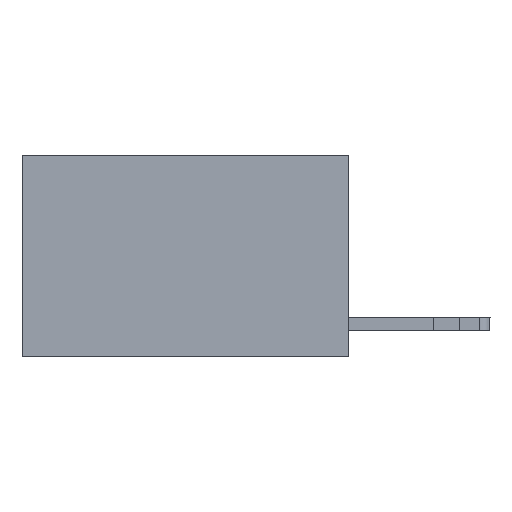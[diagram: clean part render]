
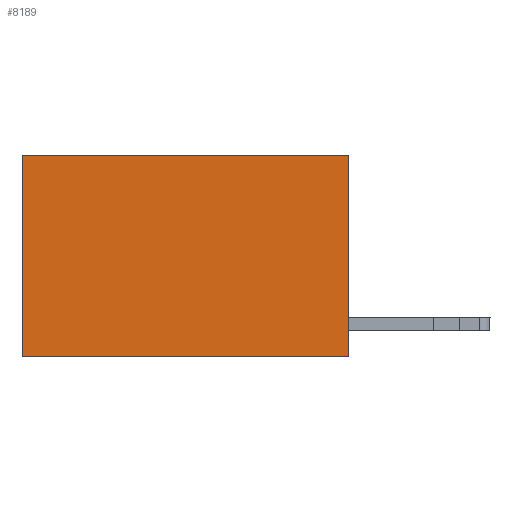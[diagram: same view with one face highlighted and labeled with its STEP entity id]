
A CAD part, left-side view. The second image highlights one B-rep face of the part: STEP entity #8189.
In plain terms, the highlighted planar face has unit normal (-1, 0, 0).
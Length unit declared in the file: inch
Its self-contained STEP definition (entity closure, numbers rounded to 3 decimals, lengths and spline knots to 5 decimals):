
#382 = DIRECTION ( 'NONE',  ( 0., 1., 0. ) ) ;
#723 = CARTESIAN_POINT ( 'NONE',  ( 0.2625, 0., -0.37 ) ) ;
#1535 = CARTESIAN_POINT ( 'NONE',  ( 0.2625, 0.6, 0. ) ) ;
#2371 = ORIENTED_EDGE ( 'NONE', *, *, #15071, .F. ) ;
#3577 = LINE ( 'NONE', #22422, #19623 ) ;
#3812 = VERTEX_POINT ( 'NONE', #4313 ) ;
#4313 = CARTESIAN_POINT ( 'NONE',  ( 0.2625, 0., 0. ) ) ;
#4358 = DIRECTION ( 'NONE',  ( 0., 1., 0. ) ) ;
#5028 = ORIENTED_EDGE ( 'NONE', *, *, #10811, .T. ) ;
#6705 = CARTESIAN_POINT ( 'NONE',  ( 0.2625, 0., -0.37 ) ) ;
#7108 = DIRECTION ( 'NONE',  ( 1., 0., 0. ) ) ;
#7636 = LINE ( 'NONE', #10611, #12531 ) ;
#8189 = ADVANCED_FACE ( 'NONE', ( #9752 ), #13310, .F. ) ;
#9030 = VERTEX_POINT ( 'NONE', #723 ) ;
#9297 = AXIS2_PLACEMENT_3D ( 'NONE', #19613, #7108, #21728 ) ;
#9409 = LINE ( 'NONE', #17006, #25422 ) ;
#9752 = FACE_OUTER_BOUND ( 'NONE', #26783, .T. ) ;
#10611 = CARTESIAN_POINT ( 'NONE',  ( 0.2625, 0., 0. ) ) ;
#10811 = EDGE_CURVE ( 'NONE', #3812, #16373, #7636, .T. ) ;
#12128 = VERTEX_POINT ( 'NONE', #17980 ) ;
#12531 = VECTOR ( 'NONE', #4358, 39.37008 ) ;
#13310 = PLANE ( 'NONE',  #9297 ) ;
#15071 = EDGE_CURVE ( 'NONE', #3812, #9030, #3577, .T. ) ;
#16373 = VERTEX_POINT ( 'NONE', #1535 ) ;
#16579 = EDGE_CURVE ( 'NONE', #16373, #12128, #9409, .T. ) ;
#17006 = CARTESIAN_POINT ( 'NONE',  ( 0.2625, 0.6, 0. ) ) ;
#17344 = ORIENTED_EDGE ( 'NONE', *, *, #21654, .F. ) ;
#17980 = CARTESIAN_POINT ( 'NONE',  ( 0.2625, 0.6, -0.37 ) ) ;
#19123 = DIRECTION ( 'NONE',  ( 0., 0., -1. ) ) ;
#19613 = CARTESIAN_POINT ( 'NONE',  ( 0.2625, 0., 0. ) ) ;
#19623 = VECTOR ( 'NONE', #26592, 39.37008 ) ;
#20960 = VECTOR ( 'NONE', #382, 39.37008 ) ;
#21618 = LINE ( 'NONE', #6705, #20960 ) ;
#21654 = EDGE_CURVE ( 'NONE', #9030, #12128, #21618, .T. ) ;
#21728 = DIRECTION ( 'NONE',  ( 0., 0., -1. ) ) ;
#22422 = CARTESIAN_POINT ( 'NONE',  ( 0.2625, 0., 0. ) ) ;
#25422 = VECTOR ( 'NONE', #19123, 39.37008 ) ;
#26592 = DIRECTION ( 'NONE',  ( 0., 0., -1. ) ) ;
#26783 = EDGE_LOOP ( 'NONE', ( #27097, #17344, #2371, #5028 ) ) ;
#27097 = ORIENTED_EDGE ( 'NONE', *, *, #16579, .T. ) ;
